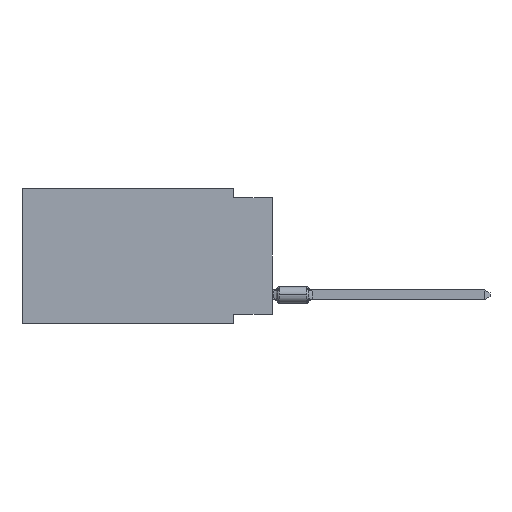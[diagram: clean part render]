
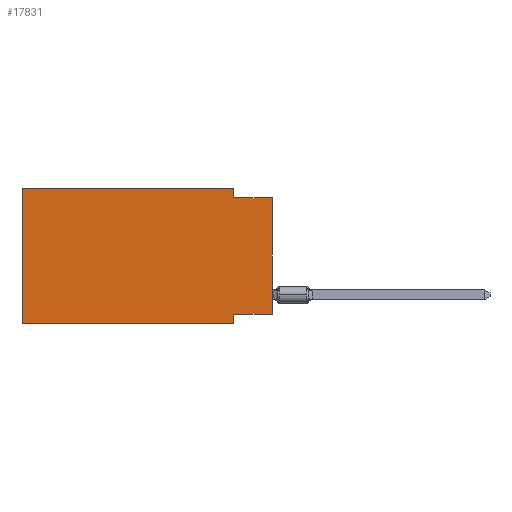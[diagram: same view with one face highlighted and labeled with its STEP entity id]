
A CAD part, left-side view. The second image highlights one B-rep face of the part: STEP entity #17831.
In plain terms, the highlighted planar face has unit normal (-1, 0, 0).
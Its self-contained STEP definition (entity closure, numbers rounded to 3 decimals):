
#7 = CARTESIAN_POINT ( 'NONE',  ( 0., 16.383, -8.89 ) ) ;
#333 = VECTOR ( 'NONE', #4800, 1000. ) ;
#361 = AXIS2_PLACEMENT_3D ( 'NONE', #20921, #5251, #3035 ) ;
#631 = CARTESIAN_POINT ( 'NONE',  ( 0., 0., -8.255 ) ) ;
#668 = DIRECTION ( 'NONE',  ( 0., -1., 0. ) ) ;
#2234 = VECTOR ( 'NONE', #15832, 1000. ) ;
#2559 = DIRECTION ( 'NONE',  ( 0., 0., -1. ) ) ;
#2822 = LINE ( 'NONE', #10788, #25268 ) ;
#3035 = DIRECTION ( 'NONE',  ( 0., 0., -1. ) ) ;
#3421 = VERTEX_POINT ( 'NONE', #3761 ) ;
#3761 = CARTESIAN_POINT ( 'NONE',  ( 0., 0., -0.635 ) ) ;
#3762 = ORIENTED_EDGE ( 'NONE', *, *, #14575, .T. ) ;
#4800 = DIRECTION ( 'NONE',  ( 0., 1., 0. ) ) ;
#5204 = VECTOR ( 'NONE', #16885, 1000. ) ;
#5251 = DIRECTION ( 'NONE',  ( 1., 0., 0. ) ) ;
#5279 = CARTESIAN_POINT ( 'NONE',  ( 0., 2.54, 0. ) ) ;
#5282 = LINE ( 'NONE', #14830, #16193 ) ;
#5605 = VECTOR ( 'NONE', #668, 1000. ) ;
#5742 = VERTEX_POINT ( 'NONE', #5279 ) ;
#5832 = ORIENTED_EDGE ( 'NONE', *, *, #17432, .F. ) ;
#6265 = EDGE_CURVE ( 'NONE', #20087, #23752, #13746, .T. ) ;
#6455 = ORIENTED_EDGE ( 'NONE', *, *, #9794, .F. ) ;
#6814 = CARTESIAN_POINT ( 'NONE',  ( 0., 0., -8.255 ) ) ;
#8247 = ORIENTED_EDGE ( 'NONE', *, *, #23453, .T. ) ;
#8364 = LINE ( 'NONE', #18571, #5605 ) ;
#8650 = CARTESIAN_POINT ( 'NONE',  ( 0., 2.54, -0.635 ) ) ;
#8798 = DIRECTION ( 'NONE',  ( 0., -1., 0. ) ) ;
#9755 = EDGE_CURVE ( 'NONE', #19529, #17043, #17092, .T. ) ;
#9794 = EDGE_CURVE ( 'NONE', #17043, #5742, #8364, .T. ) ;
#10464 = DIRECTION ( 'NONE',  ( 0., 0., 1. ) ) ;
#10788 = CARTESIAN_POINT ( 'NONE',  ( 0., 16.383, -8.89 ) ) ;
#12472 = VECTOR ( 'NONE', #2559, 1000. ) ;
#12597 = LINE ( 'NONE', #14448, #12472 ) ;
#12956 = LINE ( 'NONE', #20920, #5204 ) ;
#12957 = PLANE ( 'NONE',  #361 ) ;
#13209 = ORIENTED_EDGE ( 'NONE', *, *, #9755, .F. ) ;
#13746 = LINE ( 'NONE', #25624, #2234 ) ;
#14448 = CARTESIAN_POINT ( 'NONE',  ( 0., 2.54, 0. ) ) ;
#14575 = EDGE_CURVE ( 'NONE', #19529, #23752, #2822, .T. ) ;
#14812 = VECTOR ( 'NONE', #10464, 1000. ) ;
#14830 = CARTESIAN_POINT ( 'NONE',  ( 0., 0., -0.635 ) ) ;
#15059 = FACE_OUTER_BOUND ( 'NONE', #25649, .T. ) ;
#15832 = DIRECTION ( 'NONE',  ( 0., 0., -1. ) ) ;
#16193 = VECTOR ( 'NONE', #20714, 1000. ) ;
#16434 = CARTESIAN_POINT ( 'NONE',  ( 0., 2.54, -8.89 ) ) ;
#16885 = DIRECTION ( 'NONE',  ( 0., 0., 1. ) ) ;
#17043 = VERTEX_POINT ( 'NONE', #17337 ) ;
#17092 = LINE ( 'NONE', #20276, #14812 ) ;
#17337 = CARTESIAN_POINT ( 'NONE',  ( 0., 16.383, 0. ) ) ;
#17356 = ORIENTED_EDGE ( 'NONE', *, *, #22391, .F. ) ;
#17432 = EDGE_CURVE ( 'NONE', #18778, #3421, #5282, .T. ) ;
#17759 = ORIENTED_EDGE ( 'NONE', *, *, #19888, .F. ) ;
#17831 = ADVANCED_FACE ( 'NONE', ( #15059 ), #12957, .F. ) ;
#18571 = CARTESIAN_POINT ( 'NONE',  ( 0., 16.383, 0. ) ) ;
#18678 = LINE ( 'NONE', #631, #333 ) ;
#18763 = ORIENTED_EDGE ( 'NONE', *, *, #6265, .F. ) ;
#18778 = VERTEX_POINT ( 'NONE', #8650 ) ;
#19529 = VERTEX_POINT ( 'NONE', #7 ) ;
#19888 = EDGE_CURVE ( 'NONE', #5742, #18778, #12597, .T. ) ;
#20087 = VERTEX_POINT ( 'NONE', #23707 ) ;
#20276 = CARTESIAN_POINT ( 'NONE',  ( 0., 16.383, 0. ) ) ;
#20714 = DIRECTION ( 'NONE',  ( 0., -1., 0. ) ) ;
#20920 = CARTESIAN_POINT ( 'NONE',  ( 0., 0., 0. ) ) ;
#20921 = CARTESIAN_POINT ( 'NONE',  ( 0., 16.383, 0. ) ) ;
#22391 = EDGE_CURVE ( 'NONE', #24685, #20087, #18678, .T. ) ;
#23453 = EDGE_CURVE ( 'NONE', #24685, #3421, #12956, .T. ) ;
#23707 = CARTESIAN_POINT ( 'NONE',  ( 0., 2.54, -8.255 ) ) ;
#23752 = VERTEX_POINT ( 'NONE', #16434 ) ;
#24685 = VERTEX_POINT ( 'NONE', #6814 ) ;
#25268 = VECTOR ( 'NONE', #8798, 1000. ) ;
#25624 = CARTESIAN_POINT ( 'NONE',  ( 0., 2.54, -8.89 ) ) ;
#25649 = EDGE_LOOP ( 'NONE', ( #8247, #5832, #17759, #6455, #13209, #3762, #18763, #17356 ) ) ;
